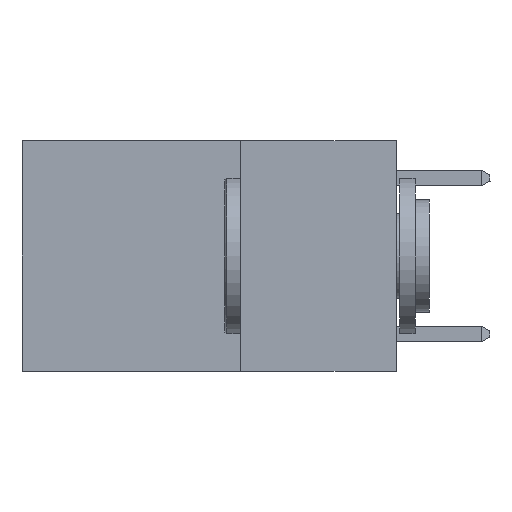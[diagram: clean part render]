
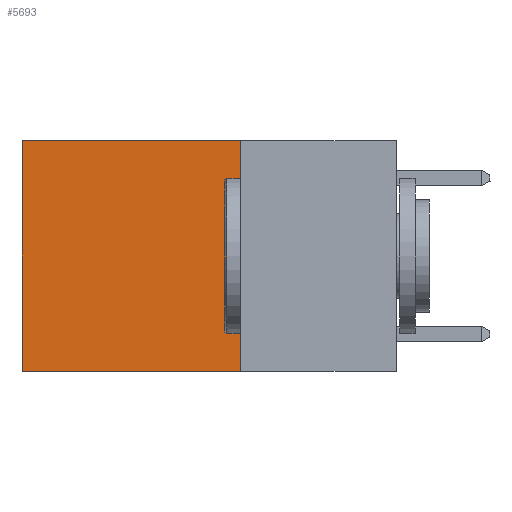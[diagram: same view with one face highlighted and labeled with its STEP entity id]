
A CAD part, left-side view. The second image highlights one B-rep face of the part: STEP entity #5693.
In plain terms, the highlighted planar face has unit normal (-1, 0, 0).
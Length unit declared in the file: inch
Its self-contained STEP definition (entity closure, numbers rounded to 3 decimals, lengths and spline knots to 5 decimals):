
#22 = LINE ( 'NONE', #15283, #11049 ) ;
#1675 = CARTESIAN_POINT ( 'NONE',  ( 0.2625, 0.25, 0. ) ) ;
#2287 = EDGE_CURVE ( 'NONE', #17422, #15180, #18468, .T. ) ;
#3001 = VERTEX_POINT ( 'NONE', #7704 ) ;
#3615 = EDGE_CURVE ( 'NONE', #13710, #15180, #22, .T. ) ;
#3825 = CARTESIAN_POINT ( 'NONE',  ( 0.2625, 0.6, -0.37 ) ) ;
#5161 = DIRECTION ( 'NONE',  ( 0., 1., 0. ) ) ;
#5511 = CARTESIAN_POINT ( 'NONE',  ( 0.2625, 0.25, -0.37 ) ) ;
#5693 = ADVANCED_FACE ( 'NONE', ( #9816 ), #17577, .F. ) ;
#6433 = DIRECTION ( 'NONE',  ( 0., 0., -1. ) ) ;
#6595 = LINE ( 'NONE', #1675, #17336 ) ;
#6845 = DIRECTION ( 'NONE',  ( 0., 0., -1. ) ) ;
#7704 = CARTESIAN_POINT ( 'NONE',  ( 0.2625, 0.25, 0. ) ) ;
#7884 = CARTESIAN_POINT ( 'NONE',  ( 0.2625, 0.6, 0. ) ) ;
#8542 = VECTOR ( 'NONE', #17139, 39.37008 ) ;
#8997 = LINE ( 'NONE', #15755, #8542 ) ;
#9363 = EDGE_CURVE ( 'NONE', #3001, #17422, #6595, .T. ) ;
#9816 = FACE_OUTER_BOUND ( 'NONE', #12976, .T. ) ;
#10084 = ORIENTED_EDGE ( 'NONE', *, *, #18473, .T. ) ;
#10218 = ORIENTED_EDGE ( 'NONE', *, *, #2287, .F. ) ;
#11049 = VECTOR ( 'NONE', #6845, 39.37008 ) ;
#11264 = ORIENTED_EDGE ( 'NONE', *, *, #3615, .T. ) ;
#11489 = AXIS2_PLACEMENT_3D ( 'NONE', #12044, #14867, #6433 ) ;
#11496 = ORIENTED_EDGE ( 'NONE', *, *, #9363, .F. ) ;
#12044 = CARTESIAN_POINT ( 'NONE',  ( 0.2625, 0.25, 0. ) ) ;
#12976 = EDGE_LOOP ( 'NONE', ( #11264, #10218, #11496, #10084 ) ) ;
#13649 = CARTESIAN_POINT ( 'NONE',  ( 0.2625, 0.25, -0.37 ) ) ;
#13710 = VERTEX_POINT ( 'NONE', #7884 ) ;
#14867 = DIRECTION ( 'NONE',  ( 1., 0., 0. ) ) ;
#15180 = VERTEX_POINT ( 'NONE', #3825 ) ;
#15273 = VECTOR ( 'NONE', #5161, 39.37008 ) ;
#15283 = CARTESIAN_POINT ( 'NONE',  ( 0.2625, 0.6, 0. ) ) ;
#15755 = CARTESIAN_POINT ( 'NONE',  ( 0.2625, 0.25, 0. ) ) ;
#17139 = DIRECTION ( 'NONE',  ( 0., 1., 0. ) ) ;
#17336 = VECTOR ( 'NONE', #17638, 39.37008 ) ;
#17422 = VERTEX_POINT ( 'NONE', #13649 ) ;
#17577 = PLANE ( 'NONE',  #11489 ) ;
#17638 = DIRECTION ( 'NONE',  ( 0., 0., -1. ) ) ;
#18468 = LINE ( 'NONE', #5511, #15273 ) ;
#18473 = EDGE_CURVE ( 'NONE', #3001, #13710, #8997, .T. ) ;
